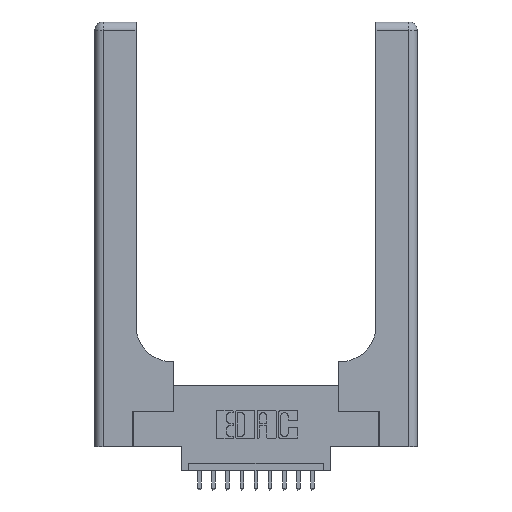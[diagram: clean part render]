
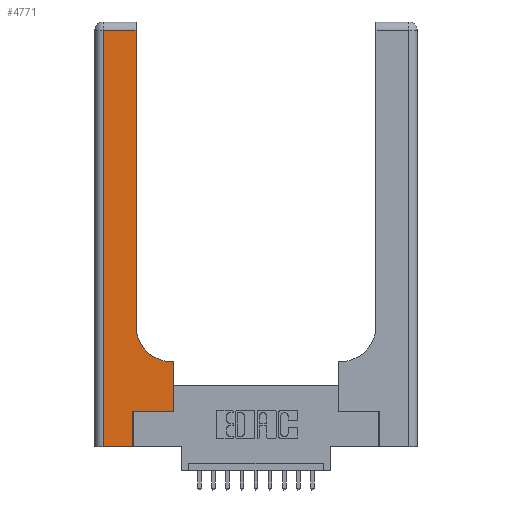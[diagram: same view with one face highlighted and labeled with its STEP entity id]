
A CAD part, top view. The second image highlights one B-rep face of the part: STEP entity #4771.
In plain terms, the highlighted planar face has unit normal (0, 0, 1).
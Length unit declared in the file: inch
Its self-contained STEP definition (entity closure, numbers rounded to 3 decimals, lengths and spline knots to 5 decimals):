
#368 = ORIENTED_EDGE ( 'NONE', *, *, #4831, .T. ) ;
#659 = VERTEX_POINT ( 'NONE', #7223 ) ;
#739 = CARTESIAN_POINT ( 'NONE',  ( 0.06, 2.94, 0.37 ) ) ;
#928 = CARTESIAN_POINT ( 'NONE',  ( 0.5415, 0.6, 0.37 ) ) ;
#1838 = EDGE_CURVE ( 'NONE', #6813, #8154, #7318, .T. ) ;
#2185 = VERTEX_POINT ( 'NONE', #739 ) ;
#2953 = CARTESIAN_POINT ( 'NONE',  ( 0.2915, 3., 0.37 ) ) ;
#2962 = CARTESIAN_POINT ( 'NONE',  ( 0.269, 0., 0.37 ) ) ;
#3185 = DIRECTION ( 'NONE',  ( -1., 0., 0. ) ) ;
#3467 = VERTEX_POINT ( 'NONE', #13342 ) ;
#3469 = EDGE_CURVE ( 'NONE', #7981, #6813, #8936, .T. ) ;
#3808 = VECTOR ( 'NONE', #5623, 39.37008 ) ;
#4224 = CARTESIAN_POINT ( 'NONE',  ( 0., 3., 0.37 ) ) ;
#4487 = DIRECTION ( 'NONE',  ( 1., 0., 0. ) ) ;
#4706 = ORIENTED_EDGE ( 'NONE', *, *, #6041, .T. ) ;
#4758 = LINE ( 'NONE', #10834, #9735 ) ;
#4771 = ADVANCED_FACE ( 'NONE', ( #14555 ), #15870, .F. ) ;
#4831 = EDGE_CURVE ( 'NONE', #8154, #3467, #11503, .T. ) ;
#5269 = DIRECTION ( 'NONE',  ( 0., 1., 0. ) ) ;
#5335 = VECTOR ( 'NONE', #10909, 39.37008 ) ;
#5410 = ORIENTED_EDGE ( 'NONE', *, *, #13951, .T. ) ;
#5533 = DIRECTION ( 'NONE',  ( 0., 0., -1. ) ) ;
#5623 = DIRECTION ( 'NONE',  ( 0., 1., 0. ) ) ;
#5849 = LINE ( 'NONE', #2962, #8823 ) ;
#6041 = EDGE_CURVE ( 'NONE', #659, #15577, #5849, .T. ) ;
#6078 = VECTOR ( 'NONE', #14703, 39.37008 ) ;
#6167 = EDGE_LOOP ( 'NONE', ( #368, #5410, #15109, #13959, #4706, #13320, #9211, #15410, #9538 ) ) ;
#6674 = CARTESIAN_POINT ( 'NONE',  ( 0.5585, 0.6, 0.37 ) ) ;
#6813 = VERTEX_POINT ( 'NONE', #928 ) ;
#6824 = DIRECTION ( 'NONE',  ( 0., 0., -1. ) ) ;
#6975 = LINE ( 'NONE', #10957, #9591 ) ;
#7203 = EDGE_CURVE ( 'NONE', #12541, #659, #11631, .T. ) ;
#7223 = CARTESIAN_POINT ( 'NONE',  ( 0.269, 0., 0.37 ) ) ;
#7318 = CIRCLE ( 'NONE', #16410, 0.25 ) ;
#7678 = EDGE_CURVE ( 'NONE', #15577, #7949, #6975, .T. ) ;
#7949 = VERTEX_POINT ( 'NONE', #11363 ) ;
#7981 = VERTEX_POINT ( 'NONE', #6674 ) ;
#8154 = VERTEX_POINT ( 'NONE', #13826 ) ;
#8567 = LINE ( 'NONE', #13438, #3808 ) ;
#8823 = VECTOR ( 'NONE', #5269, 39.37008 ) ;
#8936 = LINE ( 'NONE', #13401, #5335 ) ;
#8959 = VECTOR ( 'NONE', #15885, 39.37008 ) ;
#9198 = VECTOR ( 'NONE', #10283, 39.37008 ) ;
#9211 = ORIENTED_EDGE ( 'NONE', *, *, #12289, .T. ) ;
#9538 = ORIENTED_EDGE ( 'NONE', *, *, #1838, .T. ) ;
#9591 = VECTOR ( 'NONE', #4487, 39.37008 ) ;
#9623 = CARTESIAN_POINT ( 'NONE',  ( 0., 2.94, 0.37 ) ) ;
#9735 = VECTOR ( 'NONE', #15851, 39.37008 ) ;
#10114 = CARTESIAN_POINT ( 'NONE',  ( 0.06, 0., 0.37 ) ) ;
#10228 = CARTESIAN_POINT ( 'NONE',  ( 0.269, 0.25, 0.37 ) ) ;
#10283 = DIRECTION ( 'NONE',  ( 1., 0., 0. ) ) ;
#10834 = CARTESIAN_POINT ( 'NONE',  ( 0.06, 3., 0.37 ) ) ;
#10909 = DIRECTION ( 'NONE',  ( -1., 0., 0. ) ) ;
#10957 = CARTESIAN_POINT ( 'NONE',  ( 0.269, 0.25, 0.37 ) ) ;
#11040 = AXIS2_PLACEMENT_3D ( 'NONE', #4224, #5533, #3185 ) ;
#11363 = CARTESIAN_POINT ( 'NONE',  ( 0.5585, 0.25, 0.37 ) ) ;
#11503 = LINE ( 'NONE', #2953, #6078 ) ;
#11631 = LINE ( 'NONE', #14071, #9198 ) ;
#12289 = EDGE_CURVE ( 'NONE', #7949, #7981, #8567, .T. ) ;
#12541 = VERTEX_POINT ( 'NONE', #10114 ) ;
#13191 = CARTESIAN_POINT ( 'NONE',  ( 0.5415, 0.85, 0.37 ) ) ;
#13320 = ORIENTED_EDGE ( 'NONE', *, *, #7678, .T. ) ;
#13342 = CARTESIAN_POINT ( 'NONE',  ( 0.2915, 2.94, 0.37 ) ) ;
#13400 = LINE ( 'NONE', #9623, #8959 ) ;
#13401 = CARTESIAN_POINT ( 'NONE',  ( 0.2915, 0.6, 0.37 ) ) ;
#13438 = CARTESIAN_POINT ( 'NONE',  ( 0.5585, 0.25, 0.37 ) ) ;
#13826 = CARTESIAN_POINT ( 'NONE',  ( 0.2915, 0.85, 0.37 ) ) ;
#13951 = EDGE_CURVE ( 'NONE', #3467, #2185, #13400, .T. ) ;
#13959 = ORIENTED_EDGE ( 'NONE', *, *, #7203, .T. ) ;
#14071 = CARTESIAN_POINT ( 'NONE',  ( 0., 0., 0.37 ) ) ;
#14555 = FACE_OUTER_BOUND ( 'NONE', #6167, .T. ) ;
#14566 = EDGE_CURVE ( 'NONE', #2185, #12541, #4758, .T. ) ;
#14703 = DIRECTION ( 'NONE',  ( 0., 1., 0. ) ) ;
#15109 = ORIENTED_EDGE ( 'NONE', *, *, #14566, .T. ) ;
#15410 = ORIENTED_EDGE ( 'NONE', *, *, #3469, .T. ) ;
#15577 = VERTEX_POINT ( 'NONE', #10228 ) ;
#15717 = DIRECTION ( 'NONE',  ( 1., 0., 0. ) ) ;
#15851 = DIRECTION ( 'NONE',  ( 0., -1., 0. ) ) ;
#15870 = PLANE ( 'NONE',  #11040 ) ;
#15885 = DIRECTION ( 'NONE',  ( -1., 0., 0. ) ) ;
#16410 = AXIS2_PLACEMENT_3D ( 'NONE', #13191, #6824, #15717 ) ;
